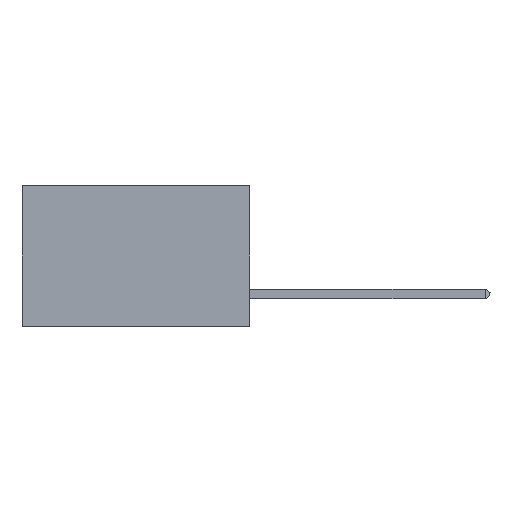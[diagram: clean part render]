
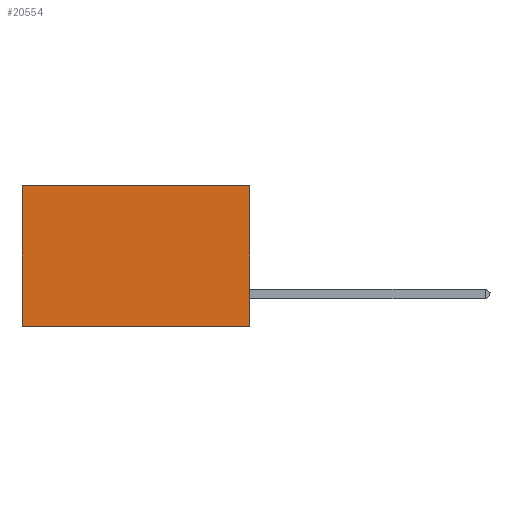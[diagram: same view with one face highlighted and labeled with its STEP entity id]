
A CAD part, left-side view. The second image highlights one B-rep face of the part: STEP entity #20554.
In plain terms, the highlighted planar face has unit normal (-1, 0, 0).
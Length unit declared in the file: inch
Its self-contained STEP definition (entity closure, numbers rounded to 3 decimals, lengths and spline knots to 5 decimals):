
#956 = ORIENTED_EDGE ( 'NONE', *, *, #23082, .F. ) ;
#1117 = LINE ( 'NONE', #5490, #29668 ) ;
#2931 = VECTOR ( 'NONE', #25106, 39.37008 ) ;
#4637 = ORIENTED_EDGE ( 'NONE', *, *, #5283, .T. ) ;
#5283 = EDGE_CURVE ( 'NONE', #32961, #5968, #8409, .T. ) ;
#5490 = CARTESIAN_POINT ( 'NONE',  ( 0.2875, 0., 0. ) ) ;
#5968 = VERTEX_POINT ( 'NONE', #25013 ) ;
#6429 = FACE_OUTER_BOUND ( 'NONE', #22505, .T. ) ;
#7607 = VECTOR ( 'NONE', #25841, 39.37008 ) ;
#8409 = LINE ( 'NONE', #25051, #7607 ) ;
#13743 = VERTEX_POINT ( 'NONE', #26848 ) ;
#15624 = EDGE_CURVE ( 'NONE', #5968, #19209, #23023, .T. ) ;
#18087 = EDGE_CURVE ( 'NONE', #32961, #13743, #1117, .T. ) ;
#19209 = VERTEX_POINT ( 'NONE', #25773 ) ;
#19583 = LINE ( 'NONE', #32518, #29665 ) ;
#20376 = DIRECTION ( 'NONE',  ( 0., 0., -1. ) ) ;
#20554 = ADVANCED_FACE ( 'NONE', ( #6429 ), #20591, .F. ) ;
#20591 = PLANE ( 'NONE',  #32910 ) ;
#22505 = EDGE_LOOP ( 'NONE', ( #30230, #956, #24316, #4637 ) ) ;
#22552 = DIRECTION ( 'NONE',  ( 0., 0., -1. ) ) ;
#23023 = LINE ( 'NONE', #33013, #2931 ) ;
#23082 = EDGE_CURVE ( 'NONE', #13743, #19209, #19583, .T. ) ;
#24316 = ORIENTED_EDGE ( 'NONE', *, *, #18087, .F. ) ;
#25013 = CARTESIAN_POINT ( 'NONE',  ( 0.2875, 0.6, 0. ) ) ;
#25051 = CARTESIAN_POINT ( 'NONE',  ( 0.2875, 0., 0. ) ) ;
#25106 = DIRECTION ( 'NONE',  ( 0., 0., -1. ) ) ;
#25458 = DIRECTION ( 'NONE',  ( 1., 0., 0. ) ) ;
#25773 = CARTESIAN_POINT ( 'NONE',  ( 0.2875, 0.6, -0.37 ) ) ;
#25841 = DIRECTION ( 'NONE',  ( 0., 1., 0. ) ) ;
#26848 = CARTESIAN_POINT ( 'NONE',  ( 0.2875, 0., -0.37 ) ) ;
#27642 = DIRECTION ( 'NONE',  ( 0., 1., 0. ) ) ;
#28257 = CARTESIAN_POINT ( 'NONE',  ( 0.2875, 0., 0. ) ) ;
#29665 = VECTOR ( 'NONE', #27642, 39.37008 ) ;
#29668 = VECTOR ( 'NONE', #22552, 39.37008 ) ;
#30230 = ORIENTED_EDGE ( 'NONE', *, *, #15624, .T. ) ;
#31967 = CARTESIAN_POINT ( 'NONE',  ( 0.2875, 0., 0. ) ) ;
#32518 = CARTESIAN_POINT ( 'NONE',  ( 0.2875, 0., -0.37 ) ) ;
#32910 = AXIS2_PLACEMENT_3D ( 'NONE', #28257, #25458, #20376 ) ;
#32961 = VERTEX_POINT ( 'NONE', #31967 ) ;
#33013 = CARTESIAN_POINT ( 'NONE',  ( 0.2875, 0.6, 0. ) ) ;
